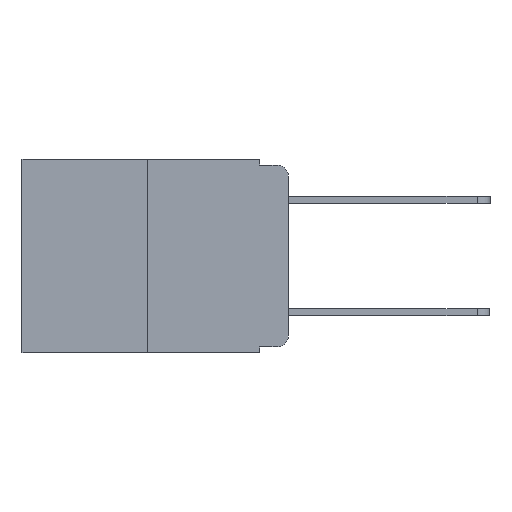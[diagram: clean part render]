
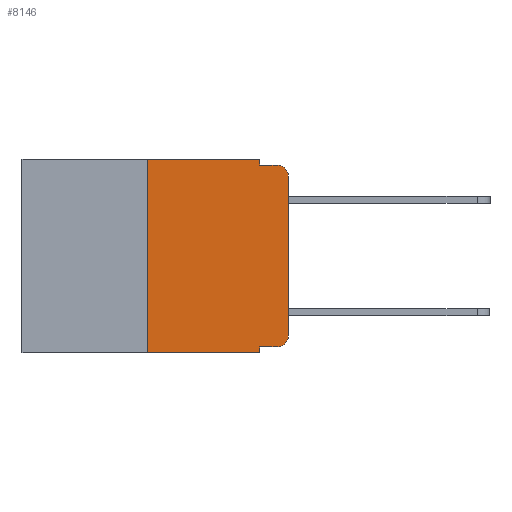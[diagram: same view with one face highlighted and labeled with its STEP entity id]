
A CAD part, left-side view. The second image highlights one B-rep face of the part: STEP entity #8146.
In plain terms, the highlighted planar face has unit normal (-1, 0, 0).
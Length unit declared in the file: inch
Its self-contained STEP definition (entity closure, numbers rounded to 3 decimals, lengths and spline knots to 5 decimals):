
#62 = ORIENTED_EDGE ( 'NONE', *, *, #4314, .T. ) ;
#68 = DIRECTION ( 'NONE',  ( 0., 0., 1. ) ) ;
#107 = CARTESIAN_POINT ( 'NONE',  ( 0., 0.051, -0.333 ) ) ;
#203 = EDGE_CURVE ( 'NONE', #778, #19316, #18545, .T. ) ;
#488 = VERTEX_POINT ( 'NONE', #1766 ) ;
#767 = CARTESIAN_POINT ( 'NONE',  ( 0., 0., 0. ) ) ;
#778 = VERTEX_POINT ( 'NONE', #9823 ) ;
#799 = VERTEX_POINT ( 'NONE', #15215 ) ;
#1758 = LINE ( 'NONE', #11871, #10265 ) ;
#1766 = CARTESIAN_POINT ( 'NONE',  ( 0., 0.051, 0. ) ) ;
#2610 = DIRECTION ( 'NONE',  ( -1., 0., 0. ) ) ;
#2654 = VERTEX_POINT ( 'NONE', #12605 ) ;
#2772 = VERTEX_POINT ( 'NONE', #10367 ) ;
#3301 = CARTESIAN_POINT ( 'NONE',  ( 0., 0.473, 0. ) ) ;
#3916 = CARTESIAN_POINT ( 'NONE',  ( 0., 0.25, 0. ) ) ;
#4285 = CARTESIAN_POINT ( 'NONE',  ( 0., 0., -0.03 ) ) ;
#4314 = EDGE_CURVE ( 'NONE', #799, #778, #16352, .T. ) ;
#4519 = LINE ( 'NONE', #18573, #20610 ) ;
#5034 = DIRECTION ( 'NONE',  ( 0., -1., 0. ) ) ;
#5279 = DIRECTION ( 'NONE',  ( 0., 0., -1. ) ) ;
#5451 = LINE ( 'NONE', #3301, #9404 ) ;
#5502 = EDGE_CURVE ( 'NONE', #11586, #799, #12576, .T. ) ;
#5508 = PLANE ( 'NONE',  #12736 ) ;
#5662 = DIRECTION ( 'NONE',  ( 0., 0., 1. ) ) ;
#5822 = VERTEX_POINT ( 'NONE', #14784 ) ;
#5823 = EDGE_CURVE ( 'NONE', #15672, #488, #5451, .T. ) ;
#6050 = CARTESIAN_POINT ( 'NONE',  ( 0., 0.051, 0. ) ) ;
#7091 = EDGE_CURVE ( 'NONE', #2654, #2772, #4519, .T. ) ;
#7757 = DIRECTION ( 'NONE',  ( 0., 0., -1. ) ) ;
#8146 = ADVANCED_FACE ( 'NONE', ( #13446 ), #5508, .F. ) ;
#8926 = EDGE_CURVE ( 'NONE', #11586, #2772, #1758, .T. ) ;
#8932 = DIRECTION ( 'NONE',  ( 1., 0., 0. ) ) ;
#9159 = LINE ( 'NONE', #19073, #12310 ) ;
#9404 = VECTOR ( 'NONE', #5034, 39.37008 ) ;
#9823 = CARTESIAN_POINT ( 'NONE',  ( 0., 0., -0.313 ) ) ;
#10043 = LINE ( 'NONE', #6050, #17157 ) ;
#10265 = VECTOR ( 'NONE', #5279, 39.37008 ) ;
#10320 = DIRECTION ( 'NONE',  ( -1., 0., 0. ) ) ;
#10367 = CARTESIAN_POINT ( 'NONE',  ( 0., 0.051, -0.343 ) ) ;
#11019 = EDGE_CURVE ( 'NONE', #2654, #15672, #18334, .T. ) ;
#11054 = DIRECTION ( 'NONE',  ( 0., -1., 0. ) ) ;
#11586 = VERTEX_POINT ( 'NONE', #107 ) ;
#11871 = CARTESIAN_POINT ( 'NONE',  ( 0., 0.051, 0. ) ) ;
#12310 = VECTOR ( 'NONE', #20504, 39.37008 ) ;
#12354 = AXIS2_PLACEMENT_3D ( 'NONE', #12524, #2610, #14106 ) ;
#12524 = CARTESIAN_POINT ( 'NONE',  ( 0., 0.02, -0.03 ) ) ;
#12576 = LINE ( 'NONE', #17301, #19586 ) ;
#12605 = CARTESIAN_POINT ( 'NONE',  ( 0., 0.25, -0.343 ) ) ;
#12736 = AXIS2_PLACEMENT_3D ( 'NONE', #18081, #8932, #19521 ) ;
#13088 = EDGE_CURVE ( 'NONE', #488, #5822, #10043, .T. ) ;
#13446 = FACE_OUTER_BOUND ( 'NONE', #15296, .T. ) ;
#13575 = VERTEX_POINT ( 'NONE', #14996 ) ;
#13656 = VECTOR ( 'NONE', #68, 39.37008 ) ;
#13919 = VECTOR ( 'NONE', #5662, 39.37008 ) ;
#14106 = DIRECTION ( 'NONE',  ( 0., 0., -1. ) ) ;
#14641 = ORIENTED_EDGE ( 'NONE', *, *, #203, .T. ) ;
#14784 = CARTESIAN_POINT ( 'NONE',  ( 0., 0.051, -0.01 ) ) ;
#14996 = CARTESIAN_POINT ( 'NONE',  ( 0., 0.02, -0.01 ) ) ;
#15060 = ORIENTED_EDGE ( 'NONE', *, *, #20056, .T. ) ;
#15197 = ORIENTED_EDGE ( 'NONE', *, *, #16147, .F. ) ;
#15215 = CARTESIAN_POINT ( 'NONE',  ( 0., 0.02, -0.333 ) ) ;
#15296 = EDGE_LOOP ( 'NONE', ( #14641, #15060, #15197, #15744, #17553, #19612, #19684, #19899, #20201, #62 ) ) ;
#15483 = DIRECTION ( 'NONE',  ( 0., -1., 0. ) ) ;
#15511 = CIRCLE ( 'NONE', #12354, 0.02 ) ;
#15672 = VERTEX_POINT ( 'NONE', #17892 ) ;
#15744 = ORIENTED_EDGE ( 'NONE', *, *, #13088, .F. ) ;
#16147 = EDGE_CURVE ( 'NONE', #5822, #13575, #9159, .T. ) ;
#16352 = CIRCLE ( 'NONE', #18676, 0.02 ) ;
#17157 = VECTOR ( 'NONE', #7757, 39.37008 ) ;
#17301 = CARTESIAN_POINT ( 'NONE',  ( 0., 0.051, -0.333 ) ) ;
#17553 = ORIENTED_EDGE ( 'NONE', *, *, #5823, .F. ) ;
#17892 = CARTESIAN_POINT ( 'NONE',  ( 0., 0.25, 0. ) ) ;
#18081 = CARTESIAN_POINT ( 'NONE',  ( 0., 0.473, 0. ) ) ;
#18334 = LINE ( 'NONE', #3916, #13919 ) ;
#18545 = LINE ( 'NONE', #767, #13656 ) ;
#18573 = CARTESIAN_POINT ( 'NONE',  ( 0., 0.473, -0.343 ) ) ;
#18676 = AXIS2_PLACEMENT_3D ( 'NONE', #19320, #10320, #20742 ) ;
#19073 = CARTESIAN_POINT ( 'NONE',  ( 0., 0.051, -0.01 ) ) ;
#19316 = VERTEX_POINT ( 'NONE', #4285 ) ;
#19320 = CARTESIAN_POINT ( 'NONE',  ( 0., 0.02, -0.313 ) ) ;
#19521 = DIRECTION ( 'NONE',  ( 0., 0., -1. ) ) ;
#19586 = VECTOR ( 'NONE', #15483, 39.37008 ) ;
#19612 = ORIENTED_EDGE ( 'NONE', *, *, #11019, .F. ) ;
#19684 = ORIENTED_EDGE ( 'NONE', *, *, #7091, .T. ) ;
#19899 = ORIENTED_EDGE ( 'NONE', *, *, #8926, .F. ) ;
#20056 = EDGE_CURVE ( 'NONE', #19316, #13575, #15511, .T. ) ;
#20201 = ORIENTED_EDGE ( 'NONE', *, *, #5502, .T. ) ;
#20504 = DIRECTION ( 'NONE',  ( 0., -1., 0. ) ) ;
#20610 = VECTOR ( 'NONE', #11054, 39.37008 ) ;
#20742 = DIRECTION ( 'NONE',  ( 0., 0., -1. ) ) ;
